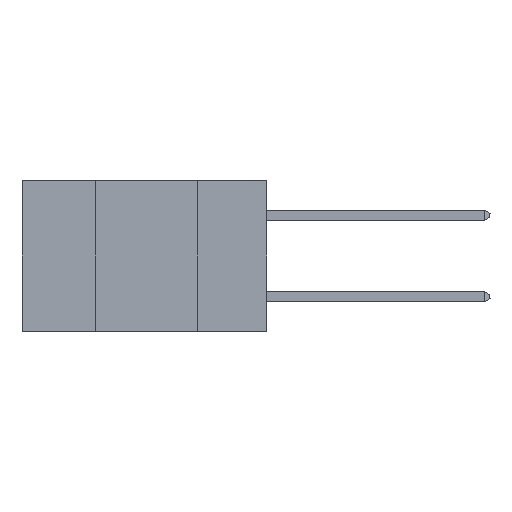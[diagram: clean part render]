
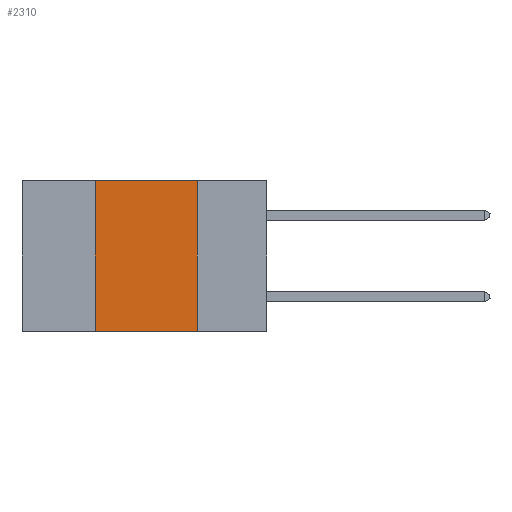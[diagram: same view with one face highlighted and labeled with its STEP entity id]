
A CAD part, left-side view. The second image highlights one B-rep face of the part: STEP entity #2310.
In plain terms, the highlighted planar face has unit normal (-1, 0, 0).
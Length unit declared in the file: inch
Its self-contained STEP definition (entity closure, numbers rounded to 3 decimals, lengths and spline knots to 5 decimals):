
#1011 = EDGE_CURVE ( 'NONE', #8757, #5317, #12477, .T. ) ;
#1212 = EDGE_LOOP ( 'NONE', ( #9962, #7807, #1603, #18347 ) ) ;
#1603 = ORIENTED_EDGE ( 'NONE', *, *, #2299, .F. ) ;
#1632 = PLANE ( 'NONE',  #7484 ) ;
#1776 = FACE_OUTER_BOUND ( 'NONE', #1212, .T. ) ;
#2299 = EDGE_CURVE ( 'NONE', #8757, #14406, #5840, .T. ) ;
#2310 = ADVANCED_FACE ( 'NONE', ( #1776 ), #1632, .F. ) ;
#2815 = LINE ( 'NONE', #8325, #10408 ) ;
#3193 = CARTESIAN_POINT ( 'NONE',  ( 0., 0.6, 0. ) ) ;
#5041 = CARTESIAN_POINT ( 'NONE',  ( 0., 0.17, -0.37 ) ) ;
#5317 = VERTEX_POINT ( 'NONE', #5041 ) ;
#5840 = LINE ( 'NONE', #10735, #13336 ) ;
#6083 = CARTESIAN_POINT ( 'NONE',  ( 0., 0.42, 0. ) ) ;
#6230 = DIRECTION ( 'NONE',  ( 0., 0., -1. ) ) ;
#7484 = AXIS2_PLACEMENT_3D ( 'NONE', #3193, #15136, #6230 ) ;
#7807 = ORIENTED_EDGE ( 'NONE', *, *, #11473, .F. ) ;
#7999 = CARTESIAN_POINT ( 'NONE',  ( 0., 0.6, 0. ) ) ;
#8325 = CARTESIAN_POINT ( 'NONE',  ( 0., 0.17, 0. ) ) ;
#8757 = VERTEX_POINT ( 'NONE', #12821 ) ;
#9828 = DIRECTION ( 'NONE',  ( 0., 0., -1. ) ) ;
#9962 = ORIENTED_EDGE ( 'NONE', *, *, #17126, .F. ) ;
#10408 = VECTOR ( 'NONE', #9828, 39.37008 ) ;
#10735 = CARTESIAN_POINT ( 'NONE',  ( 0., 0.42, 0. ) ) ;
#11154 = LINE ( 'NONE', #7999, #18848 ) ;
#11473 = EDGE_CURVE ( 'NONE', #14406, #15792, #11154, .T. ) ;
#12223 = DIRECTION ( 'NONE',  ( 0., 0., 1. ) ) ;
#12477 = LINE ( 'NONE', #13953, #19243 ) ;
#12821 = CARTESIAN_POINT ( 'NONE',  ( 0., 0.42, -0.37 ) ) ;
#13336 = VECTOR ( 'NONE', #12223, 39.37008 ) ;
#13953 = CARTESIAN_POINT ( 'NONE',  ( 0., 0.6, -0.37 ) ) ;
#14406 = VERTEX_POINT ( 'NONE', #6083 ) ;
#15136 = DIRECTION ( 'NONE',  ( 1., 0., 0. ) ) ;
#15792 = VERTEX_POINT ( 'NONE', #16839 ) ;
#16839 = CARTESIAN_POINT ( 'NONE',  ( 0., 0.17, 0. ) ) ;
#17047 = DIRECTION ( 'NONE',  ( 0., -1., 0. ) ) ;
#17126 = EDGE_CURVE ( 'NONE', #15792, #5317, #2815, .T. ) ;
#18228 = DIRECTION ( 'NONE',  ( 0., -1., 0. ) ) ;
#18347 = ORIENTED_EDGE ( 'NONE', *, *, #1011, .T. ) ;
#18848 = VECTOR ( 'NONE', #18228, 39.37008 ) ;
#19243 = VECTOR ( 'NONE', #17047, 39.37008 ) ;
